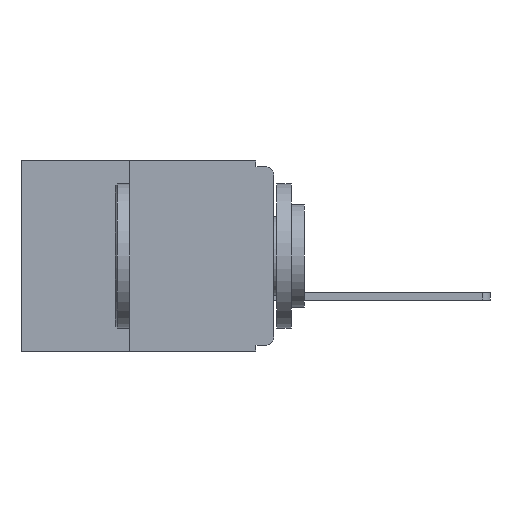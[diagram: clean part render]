
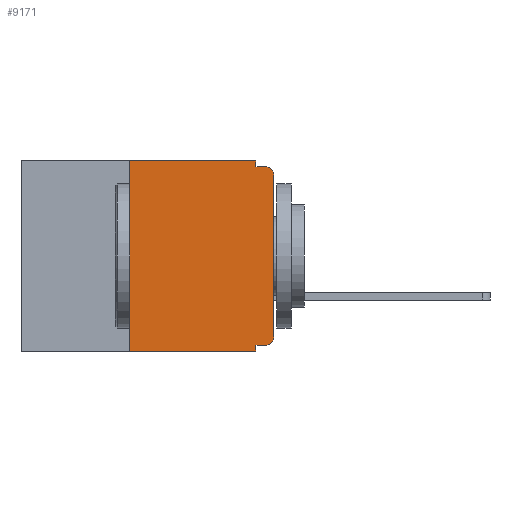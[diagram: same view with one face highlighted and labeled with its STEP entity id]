
A CAD part, left-side view. The second image highlights one B-rep face of the part: STEP entity #9171.
In plain terms, the highlighted planar face has unit normal (-1, 0, 0).
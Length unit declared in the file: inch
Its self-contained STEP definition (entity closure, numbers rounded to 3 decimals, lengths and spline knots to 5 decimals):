
#775 = EDGE_CURVE ( 'NONE', #17145, #3176, #20783, .T. ) ;
#1449 = VERTEX_POINT ( 'NONE', #11186 ) ;
#1735 = VECTOR ( 'NONE', #5475, 39.37008 ) ;
#1871 = ORIENTED_EDGE ( 'NONE', *, *, #16765, .F. ) ;
#1903 = VECTOR ( 'NONE', #6274, 39.37008 ) ;
#2270 = VECTOR ( 'NONE', #5106, 39.37008 ) ;
#2288 = LINE ( 'NONE', #6845, #1735 ) ;
#2379 = CARTESIAN_POINT ( 'NONE',  ( 0., 0., -0.025 ) ) ;
#2412 = ORIENTED_EDGE ( 'NONE', *, *, #6382, .F. ) ;
#2548 = DIRECTION ( 'NONE',  ( 0., -1., 0. ) ) ;
#2677 = EDGE_CURVE ( 'NONE', #15152, #3176, #6787, .T. ) ;
#3176 = VERTEX_POINT ( 'NONE', #18986 ) ;
#3558 = ORIENTED_EDGE ( 'NONE', *, *, #2677, .F. ) ;
#4233 = DIRECTION ( 'NONE',  ( 0., 0., -1. ) ) ;
#4237 = DIRECTION ( 'NONE',  ( 1., 0., 0. ) ) ;
#4257 = DIRECTION ( 'NONE',  ( 0., 0., 1. ) ) ;
#4378 = CARTESIAN_POINT ( 'NONE',  ( 0., 0.437, 0. ) ) ;
#4501 = CARTESIAN_POINT ( 'NONE',  ( 0., 0.25, -0.33 ) ) ;
#4699 = EDGE_CURVE ( 'NONE', #1449, #21160, #2288, .T. ) ;
#4731 = AXIS2_PLACEMENT_3D ( 'NONE', #6858, #18802, #8630 ) ;
#4769 = PLANE ( 'NONE',  #8314 ) ;
#5053 = CARTESIAN_POINT ( 'NONE',  ( 0., 0., -0.32 ) ) ;
#5096 = VERTEX_POINT ( 'NONE', #19248 ) ;
#5106 = DIRECTION ( 'NONE',  ( 0., 1., 0. ) ) ;
#5176 = DIRECTION ( 'NONE',  ( 0., -1., 0. ) ) ;
#5475 = DIRECTION ( 'NONE',  ( 0., 0., -1. ) ) ;
#5813 = VERTEX_POINT ( 'NONE', #11016 ) ;
#5817 = LINE ( 'NONE', #7088, #18942 ) ;
#6274 = DIRECTION ( 'NONE',  ( 0., -1., 0. ) ) ;
#6347 = EDGE_CURVE ( 'NONE', #6777, #15152, #20594, .T. ) ;
#6382 = EDGE_CURVE ( 'NONE', #17145, #5813, #6425, .T. ) ;
#6425 = LINE ( 'NONE', #4501, #19510 ) ;
#6777 = VERTEX_POINT ( 'NONE', #19517 ) ;
#6787 = LINE ( 'NONE', #20643, #7345 ) ;
#6845 = CARTESIAN_POINT ( 'NONE',  ( 0., 0.031, 0. ) ) ;
#6858 = CARTESIAN_POINT ( 'NONE',  ( 0., 0.015, -0.025 ) ) ;
#7088 = CARTESIAN_POINT ( 'NONE',  ( 0., 0., 0. ) ) ;
#7345 = VECTOR ( 'NONE', #21376, 39.37008 ) ;
#7898 = CARTESIAN_POINT ( 'NONE',  ( 0., 0.437, 0. ) ) ;
#8226 = VECTOR ( 'NONE', #2548, 39.37008 ) ;
#8314 = AXIS2_PLACEMENT_3D ( 'NONE', #4378, #4237, #4233 ) ;
#8537 = CARTESIAN_POINT ( 'NONE',  ( 0., 0.015, -0.305 ) ) ;
#8630 = DIRECTION ( 'NONE',  ( 0., 0., -1. ) ) ;
#8854 = DIRECTION ( 'NONE',  ( 0., 0., 1. ) ) ;
#9171 = ADVANCED_FACE ( 'NONE', ( #12499 ), #4769, .F. ) ;
#9763 = CARTESIAN_POINT ( 'NONE',  ( 0., 0.015, -0.01 ) ) ;
#9890 = EDGE_CURVE ( 'NONE', #6777, #5096, #11146, .T. ) ;
#10251 = DIRECTION ( 'NONE',  ( 0., 0., -1. ) ) ;
#11016 = CARTESIAN_POINT ( 'NONE',  ( 0., 0.25, 0. ) ) ;
#11146 = CIRCLE ( 'NONE', #22272, 0.015 ) ;
#11186 = CARTESIAN_POINT ( 'NONE',  ( 0., 0.031, 0. ) ) ;
#11359 = VERTEX_POINT ( 'NONE', #2379 ) ;
#12090 = EDGE_LOOP ( 'NONE', ( #18829, #19360, #21502, #12735, #1871, #2412, #21009, #3558, #14405, #18126 ) ) ;
#12499 = FACE_OUTER_BOUND ( 'NONE', #12090, .T. ) ;
#12735 = ORIENTED_EDGE ( 'NONE', *, *, #4699, .F. ) ;
#13265 = LINE ( 'NONE', #7898, #8226 ) ;
#13942 = CARTESIAN_POINT ( 'NONE',  ( 0., 0.437, -0.33 ) ) ;
#14405 = ORIENTED_EDGE ( 'NONE', *, *, #6347, .F. ) ;
#15152 = VERTEX_POINT ( 'NONE', #20086 ) ;
#15506 = CARTESIAN_POINT ( 'NONE',  ( 0., 0., -0.01 ) ) ;
#16429 = VECTOR ( 'NONE', #5176, 39.37008 ) ;
#16765 = EDGE_CURVE ( 'NONE', #5813, #1449, #13265, .T. ) ;
#17145 = VERTEX_POINT ( 'NONE', #20750 ) ;
#18126 = ORIENTED_EDGE ( 'NONE', *, *, #9890, .T. ) ;
#18660 = EDGE_CURVE ( 'NONE', #11359, #21897, #21082, .T. ) ;
#18717 = EDGE_CURVE ( 'NONE', #5096, #11359, #5817, .T. ) ;
#18802 = DIRECTION ( 'NONE',  ( -1., 0., 0. ) ) ;
#18829 = ORIENTED_EDGE ( 'NONE', *, *, #18717, .T. ) ;
#18942 = VECTOR ( 'NONE', #8854, 39.37008 ) ;
#18986 = CARTESIAN_POINT ( 'NONE',  ( 0., 0.031, -0.33 ) ) ;
#19248 = CARTESIAN_POINT ( 'NONE',  ( 0., 0., -0.305 ) ) ;
#19360 = ORIENTED_EDGE ( 'NONE', *, *, #18660, .T. ) ;
#19510 = VECTOR ( 'NONE', #4257, 39.37008 ) ;
#19517 = CARTESIAN_POINT ( 'NONE',  ( 0., 0.015, -0.32 ) ) ;
#20086 = CARTESIAN_POINT ( 'NONE',  ( 0., 0.031, -0.32 ) ) ;
#20433 = DIRECTION ( 'NONE',  ( -1., 0., 0. ) ) ;
#20594 = LINE ( 'NONE', #5053, #2270 ) ;
#20643 = CARTESIAN_POINT ( 'NONE',  ( 0., 0.031, -0.33 ) ) ;
#20750 = CARTESIAN_POINT ( 'NONE',  ( 0., 0.25, -0.33 ) ) ;
#20783 = LINE ( 'NONE', #13942, #1903 ) ;
#20935 = LINE ( 'NONE', #15506, #16429 ) ;
#21009 = ORIENTED_EDGE ( 'NONE', *, *, #775, .T. ) ;
#21013 = CARTESIAN_POINT ( 'NONE',  ( 0., 0.031, -0.01 ) ) ;
#21082 = CIRCLE ( 'NONE', #4731, 0.015 ) ;
#21160 = VERTEX_POINT ( 'NONE', #21013 ) ;
#21376 = DIRECTION ( 'NONE',  ( 0., 0., -1. ) ) ;
#21502 = ORIENTED_EDGE ( 'NONE', *, *, #21608, .F. ) ;
#21608 = EDGE_CURVE ( 'NONE', #21160, #21897, #20935, .T. ) ;
#21897 = VERTEX_POINT ( 'NONE', #9763 ) ;
#22272 = AXIS2_PLACEMENT_3D ( 'NONE', #8537, #20433, #10251 ) ;
